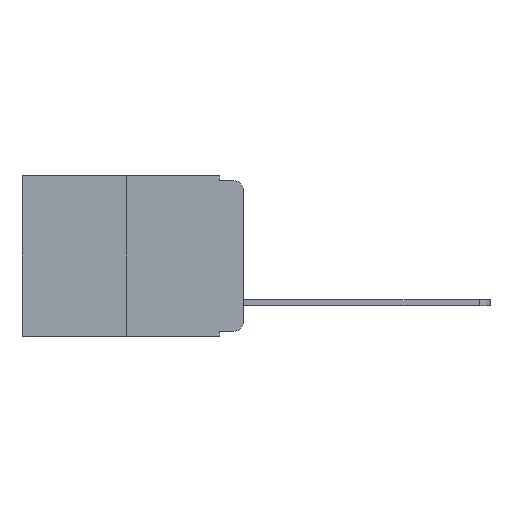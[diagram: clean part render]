
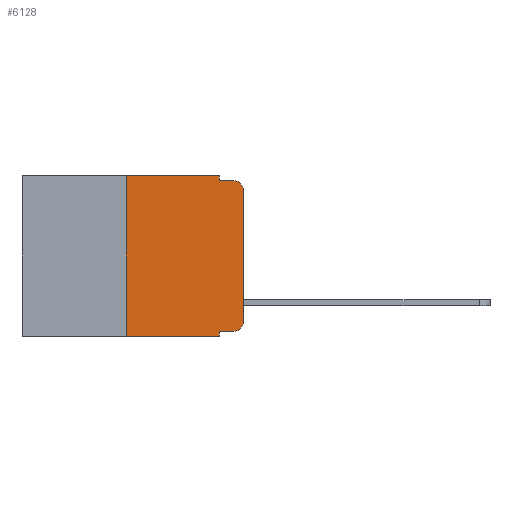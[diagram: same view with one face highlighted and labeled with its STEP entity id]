
A CAD part, left-side view. The second image highlights one B-rep face of the part: STEP entity #6128.
In plain terms, the highlighted planar face has unit normal (-1, 0, 0).
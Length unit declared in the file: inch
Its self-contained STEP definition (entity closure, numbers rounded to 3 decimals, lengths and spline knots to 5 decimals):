
#207 = ORIENTED_EDGE ( 'NONE', *, *, #5208, .T. ) ;
#245 = ORIENTED_EDGE ( 'NONE', *, *, #5628, .T. ) ;
#272 = VECTOR ( 'NONE', #7177, 39.37008 ) ;
#280 = DIRECTION ( 'NONE',  ( 0., 0., 1. ) ) ;
#335 = ORIENTED_EDGE ( 'NONE', *, *, #5164, .T. ) ;
#354 = ORIENTED_EDGE ( 'NONE', *, *, #5139, .T. ) ;
#394 = EDGE_LOOP ( 'NONE', ( #335, #207, #5948, #503, #2071, #602, #6025, #6480, #245, #354 ) ) ;
#503 = ORIENTED_EDGE ( 'NONE', *, *, #5391, .F. ) ;
#597 = CARTESIAN_POINT ( 'NONE',  ( 0., 0.051, -0.333 ) ) ;
#602 = ORIENTED_EDGE ( 'NONE', *, *, #5118, .F. ) ;
#737 = VECTOR ( 'NONE', #280, 39.37008 ) ;
#897 = CARTESIAN_POINT ( 'NONE',  ( 0., 0., -0.03 ) ) ;
#1016 = VERTEX_POINT ( 'NONE', #6100 ) ;
#1027 = VERTEX_POINT ( 'NONE', #5506 ) ;
#1102 = LINE ( 'NONE', #9433, #737 ) ;
#1107 = DIRECTION ( 'NONE',  ( 1., 0., 0. ) ) ;
#1220 = CARTESIAN_POINT ( 'NONE',  ( 0., 0.25, -0.343 ) ) ;
#1283 = VECTOR ( 'NONE', #6905, 39.37008 ) ;
#1329 = VERTEX_POINT ( 'NONE', #7999 ) ;
#1412 = LINE ( 'NONE', #597, #7555 ) ;
#2071 = ORIENTED_EDGE ( 'NONE', *, *, #2296, .F. ) ;
#2089 = VERTEX_POINT ( 'NONE', #9325 ) ;
#2139 = CARTESIAN_POINT ( 'NONE',  ( 0., 0.473, -0.343 ) ) ;
#2173 = LINE ( 'NONE', #8086, #6120 ) ;
#2296 = EDGE_CURVE ( 'NONE', #3887, #4252, #8545, .T. ) ;
#2358 = CARTESIAN_POINT ( 'NONE',  ( 0., 0.051, 0. ) ) ;
#2407 = CARTESIAN_POINT ( 'NONE',  ( 0., 0.02, -0.313 ) ) ;
#2620 = CARTESIAN_POINT ( 'NONE',  ( 0., 0.473, 0. ) ) ;
#2747 = CARTESIAN_POINT ( 'NONE',  ( 0., 0.051, -0.01 ) ) ;
#2835 = DIRECTION ( 'NONE',  ( 0., 0., -1. ) ) ;
#2861 = VECTOR ( 'NONE', #3057, 39.37008 ) ;
#2866 = CARTESIAN_POINT ( 'NONE',  ( 0., 0.051, -0.333 ) ) ;
#3057 = DIRECTION ( 'NONE',  ( 0., -1., 0. ) ) ;
#3135 = LINE ( 'NONE', #2139, #2861 ) ;
#3284 = DIRECTION ( 'NONE',  ( 0., 0., -1. ) ) ;
#3887 = VERTEX_POINT ( 'NONE', #4408 ) ;
#3977 = VERTEX_POINT ( 'NONE', #897 ) ;
#4175 = VERTEX_POINT ( 'NONE', #1220 ) ;
#4252 = VERTEX_POINT ( 'NONE', #2358 ) ;
#4408 = CARTESIAN_POINT ( 'NONE',  ( 0., 0.25, 0. ) ) ;
#4596 = AXIS2_PLACEMENT_3D ( 'NONE', #8151, #1107, #6916 ) ;
#4709 = PLANE ( 'NONE',  #4596 ) ;
#4814 = CARTESIAN_POINT ( 'NONE',  ( 0., 0.051, -0.01 ) ) ;
#5010 = EDGE_CURVE ( 'NONE', #4175, #1016, #3135, .T. ) ;
#5118 = EDGE_CURVE ( 'NONE', #4175, #3887, #1102, .T. ) ;
#5139 = EDGE_CURVE ( 'NONE', #1027, #1329, #7375, .T. ) ;
#5155 = DIRECTION ( 'NONE',  ( -1., 0., 0. ) ) ;
#5164 = EDGE_CURVE ( 'NONE', #1329, #3977, #6941, .T. ) ;
#5208 = EDGE_CURVE ( 'NONE', #3977, #2089, #6511, .T. ) ;
#5391 = EDGE_CURVE ( 'NONE', #4252, #5785, #2173, .T. ) ;
#5395 = EDGE_CURVE ( 'NONE', #5785, #2089, #5908, .T. ) ;
#5407 = EDGE_CURVE ( 'NONE', #8154, #1016, #9001, .T. ) ;
#5506 = CARTESIAN_POINT ( 'NONE',  ( 0., 0.02, -0.333 ) ) ;
#5628 = EDGE_CURVE ( 'NONE', #8154, #1027, #1412, .T. ) ;
#5785 = VERTEX_POINT ( 'NONE', #2747 ) ;
#5908 = LINE ( 'NONE', #4814, #9186 ) ;
#5948 = ORIENTED_EDGE ( 'NONE', *, *, #5395, .F. ) ;
#6025 = ORIENTED_EDGE ( 'NONE', *, *, #5010, .T. ) ;
#6100 = CARTESIAN_POINT ( 'NONE',  ( 0., 0.051, -0.343 ) ) ;
#6120 = VECTOR ( 'NONE', #2835, 39.37008 ) ;
#6128 = ADVANCED_FACE ( 'NONE', ( #9267 ), #4709, .F. ) ;
#6219 = AXIS2_PLACEMENT_3D ( 'NONE', #8988, #5155, #9515 ) ;
#6267 = AXIS2_PLACEMENT_3D ( 'NONE', #2407, #7792, #3284 ) ;
#6312 = CARTESIAN_POINT ( 'NONE',  ( 0., 0.051, 0. ) ) ;
#6480 = ORIENTED_EDGE ( 'NONE', *, *, #5407, .F. ) ;
#6511 = CIRCLE ( 'NONE', #6219, 0.02 ) ;
#6905 = DIRECTION ( 'NONE',  ( 0., 0., -1. ) ) ;
#6916 = DIRECTION ( 'NONE',  ( 0., 0., -1. ) ) ;
#6941 = LINE ( 'NONE', #8935, #8388 ) ;
#7177 = DIRECTION ( 'NONE',  ( 0., -1., 0. ) ) ;
#7375 = CIRCLE ( 'NONE', #6267, 0.02 ) ;
#7555 = VECTOR ( 'NONE', #8506, 39.37008 ) ;
#7792 = DIRECTION ( 'NONE',  ( -1., 0., 0. ) ) ;
#7999 = CARTESIAN_POINT ( 'NONE',  ( 0., 0., -0.313 ) ) ;
#8086 = CARTESIAN_POINT ( 'NONE',  ( 0., 0.051, 0. ) ) ;
#8151 = CARTESIAN_POINT ( 'NONE',  ( 0., 0.473, 0. ) ) ;
#8154 = VERTEX_POINT ( 'NONE', #2866 ) ;
#8388 = VECTOR ( 'NONE', #9477, 39.37008 ) ;
#8506 = DIRECTION ( 'NONE',  ( 0., -1., 0. ) ) ;
#8545 = LINE ( 'NONE', #2620, #272 ) ;
#8935 = CARTESIAN_POINT ( 'NONE',  ( 0., 0., 0. ) ) ;
#8988 = CARTESIAN_POINT ( 'NONE',  ( 0., 0.02, -0.03 ) ) ;
#9001 = LINE ( 'NONE', #6312, #1283 ) ;
#9186 = VECTOR ( 'NONE', #9320, 39.37008 ) ;
#9267 = FACE_OUTER_BOUND ( 'NONE', #394, .T. ) ;
#9320 = DIRECTION ( 'NONE',  ( 0., -1., 0. ) ) ;
#9325 = CARTESIAN_POINT ( 'NONE',  ( 0., 0.02, -0.01 ) ) ;
#9433 = CARTESIAN_POINT ( 'NONE',  ( 0., 0.25, 0. ) ) ;
#9477 = DIRECTION ( 'NONE',  ( 0., 0., 1. ) ) ;
#9515 = DIRECTION ( 'NONE',  ( 0., 0., -1. ) ) ;
